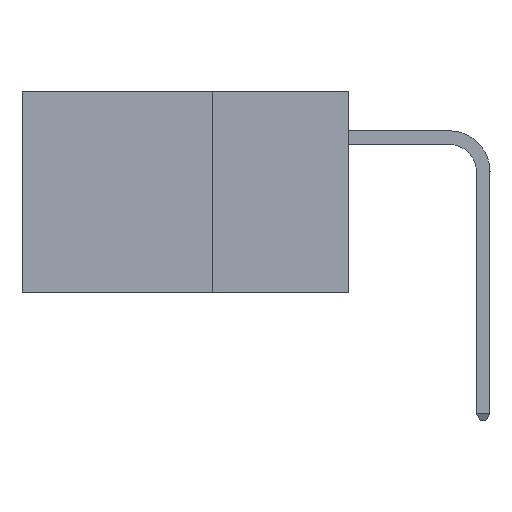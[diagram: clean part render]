
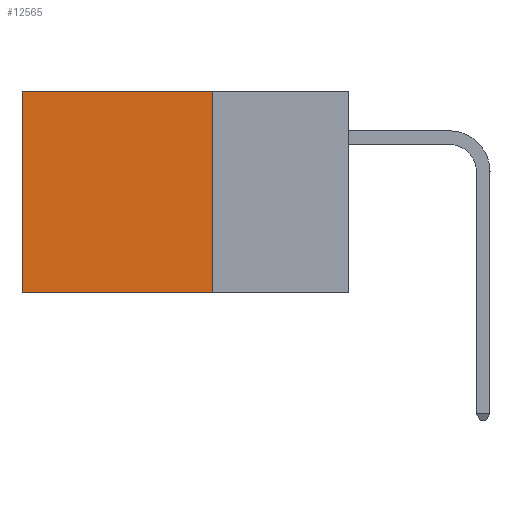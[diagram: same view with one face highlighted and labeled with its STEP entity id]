
A CAD part, left-side view. The second image highlights one B-rep face of the part: STEP entity #12565.
In plain terms, the highlighted planar face has unit normal (-1, 0, 0).
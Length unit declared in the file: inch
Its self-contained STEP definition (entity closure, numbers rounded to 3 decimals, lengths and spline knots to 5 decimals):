
#576 = ORIENTED_EDGE ( 'NONE', *, *, #17027, .F. ) ;
#1878 = VECTOR ( 'NONE', #21677, 39.37008 ) ;
#3003 = DIRECTION ( 'NONE',  ( 0., 0., -1. ) ) ;
#3564 = VECTOR ( 'NONE', #42033, 39.37008 ) ;
#3881 = EDGE_CURVE ( 'NONE', #27794, #23675, #28102, .T. ) ;
#4366 = ORIENTED_EDGE ( 'NONE', *, *, #39458, .F. ) ;
#4765 = VECTOR ( 'NONE', #15839, 39.37008 ) ;
#6282 = PLANE ( 'NONE',  #10795 ) ;
#8778 = CARTESIAN_POINT ( 'NONE',  ( 0.2875, 0.25, 0. ) ) ;
#9364 = VECTOR ( 'NONE', #3003, 39.37008 ) ;
#10795 = AXIS2_PLACEMENT_3D ( 'NONE', #17258, #41839, #44919 ) ;
#11124 = LINE ( 'NONE', #38505, #1878 ) ;
#12565 = ADVANCED_FACE ( 'NONE', ( #41594 ), #6282, .F. ) ;
#13601 = EDGE_LOOP ( 'NONE', ( #38480, #576, #4366, #41361 ) ) ;
#15839 = DIRECTION ( 'NONE',  ( 0., 0., -1. ) ) ;
#16161 = VERTEX_POINT ( 'NONE', #27500 ) ;
#17027 = EDGE_CURVE ( 'NONE', #28167, #16161, #11124, .T. ) ;
#17258 = CARTESIAN_POINT ( 'NONE',  ( 0.2875, 0.25, 0. ) ) ;
#18437 = LINE ( 'NONE', #8778, #4765 ) ;
#21677 = DIRECTION ( 'NONE',  ( 0., 1., 0. ) ) ;
#23675 = VERTEX_POINT ( 'NONE', #37301 ) ;
#27500 = CARTESIAN_POINT ( 'NONE',  ( 0.2875, 0.6, -0.37 ) ) ;
#27794 = VERTEX_POINT ( 'NONE', #35194 ) ;
#28102 = LINE ( 'NONE', #38251, #3564 ) ;
#28167 = VERTEX_POINT ( 'NONE', #33510 ) ;
#33510 = CARTESIAN_POINT ( 'NONE',  ( 0.2875, 0.25, -0.37 ) ) ;
#33928 = LINE ( 'NONE', #37805, #9364 ) ;
#35194 = CARTESIAN_POINT ( 'NONE',  ( 0.2875, 0.25, 0. ) ) ;
#37301 = CARTESIAN_POINT ( 'NONE',  ( 0.2875, 0.6, 0. ) ) ;
#37805 = CARTESIAN_POINT ( 'NONE',  ( 0.2875, 0.6, 0. ) ) ;
#38251 = CARTESIAN_POINT ( 'NONE',  ( 0.2875, 0.25, 0. ) ) ;
#38480 = ORIENTED_EDGE ( 'NONE', *, *, #39600, .T. ) ;
#38505 = CARTESIAN_POINT ( 'NONE',  ( 0.2875, 0.25, -0.37 ) ) ;
#39458 = EDGE_CURVE ( 'NONE', #27794, #28167, #18437, .T. ) ;
#39600 = EDGE_CURVE ( 'NONE', #23675, #16161, #33928, .T. ) ;
#41361 = ORIENTED_EDGE ( 'NONE', *, *, #3881, .T. ) ;
#41594 = FACE_OUTER_BOUND ( 'NONE', #13601, .T. ) ;
#41839 = DIRECTION ( 'NONE',  ( 1., 0., 0. ) ) ;
#42033 = DIRECTION ( 'NONE',  ( 0., 1., 0. ) ) ;
#44919 = DIRECTION ( 'NONE',  ( 0., 0., -1. ) ) ;
